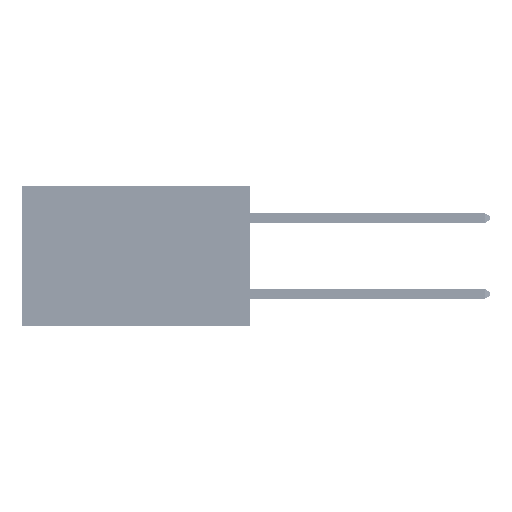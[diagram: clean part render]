
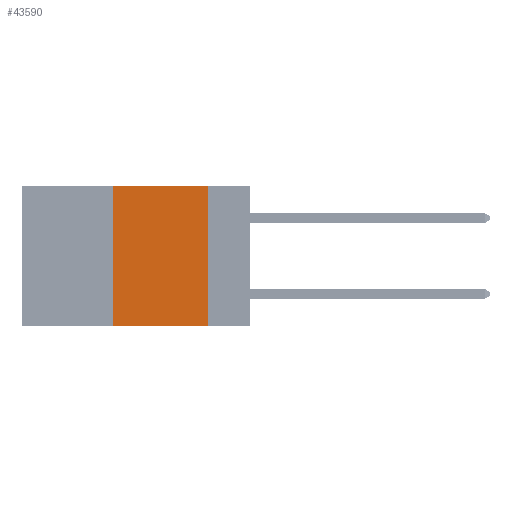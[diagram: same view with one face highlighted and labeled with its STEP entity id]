
A CAD part, left-side view. The second image highlights one B-rep face of the part: STEP entity #43590.
In plain terms, the highlighted planar face has unit normal (-1, 0, 0).
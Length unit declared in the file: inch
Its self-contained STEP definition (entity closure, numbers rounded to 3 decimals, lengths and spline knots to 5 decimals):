
#87 = VERTEX_POINT ( 'NONE', #6305 ) ;
#2628 = DIRECTION ( 'NONE',  ( 1., 0., 0. ) ) ;
#6305 = CARTESIAN_POINT ( 'NONE',  ( 0., 0.36, -0.37 ) ) ;
#7148 = LINE ( 'NONE', #38826, #11067 ) ;
#8899 = LINE ( 'NONE', #16185, #26012 ) ;
#9311 = LINE ( 'NONE', #45603, #25820 ) ;
#10166 = VERTEX_POINT ( 'NONE', #28662 ) ;
#11067 = VECTOR ( 'NONE', #35047, 39.37008 ) ;
#13826 = PLANE ( 'NONE',  #17814 ) ;
#14744 = ORIENTED_EDGE ( 'NONE', *, *, #47009, .T. ) ;
#16185 = CARTESIAN_POINT ( 'NONE',  ( 0., 0.11, 0. ) ) ;
#17814 = AXIS2_PLACEMENT_3D ( 'NONE', #18405, #2628, #21820 ) ;
#18236 = DIRECTION ( 'NONE',  ( 0., -1., 0. ) ) ;
#18269 = LINE ( 'NONE', #31185, #23751 ) ;
#18405 = CARTESIAN_POINT ( 'NONE',  ( 0., 0.6, 0. ) ) ;
#21820 = DIRECTION ( 'NONE',  ( 0., 0., -1. ) ) ;
#22657 = CARTESIAN_POINT ( 'NONE',  ( 0., 0.36, 0. ) ) ;
#22706 = CARTESIAN_POINT ( 'NONE',  ( 0., 0.11, 0. ) ) ;
#22881 = EDGE_CURVE ( 'NONE', #48929, #10166, #8899, .T. ) ;
#23751 = VECTOR ( 'NONE', #42686, 39.37008 ) ;
#25820 = VECTOR ( 'NONE', #18236, 39.37008 ) ;
#25941 = ORIENTED_EDGE ( 'NONE', *, *, #27470, .F. ) ;
#26012 = VECTOR ( 'NONE', #36666, 39.37008 ) ;
#27470 = EDGE_CURVE ( 'NONE', #87, #42415, #18269, .T. ) ;
#27716 = ORIENTED_EDGE ( 'NONE', *, *, #22881, .F. ) ;
#28662 = CARTESIAN_POINT ( 'NONE',  ( 0., 0.11, -0.37 ) ) ;
#31185 = CARTESIAN_POINT ( 'NONE',  ( 0., 0.36, 0. ) ) ;
#34156 = EDGE_LOOP ( 'NONE', ( #27716, #42161, #25941, #14744 ) ) ;
#35047 = DIRECTION ( 'NONE',  ( 0., -1., 0. ) ) ;
#36666 = DIRECTION ( 'NONE',  ( 0., 0., -1. ) ) ;
#38826 = CARTESIAN_POINT ( 'NONE',  ( 0., 0.6, -0.37 ) ) ;
#41156 = FACE_OUTER_BOUND ( 'NONE', #34156, .T. ) ;
#42161 = ORIENTED_EDGE ( 'NONE', *, *, #43551, .F. ) ;
#42415 = VERTEX_POINT ( 'NONE', #22657 ) ;
#42686 = DIRECTION ( 'NONE',  ( 0., 0., 1. ) ) ;
#43551 = EDGE_CURVE ( 'NONE', #42415, #48929, #9311, .T. ) ;
#43590 = ADVANCED_FACE ( 'NONE', ( #41156 ), #13826, .F. ) ;
#45603 = CARTESIAN_POINT ( 'NONE',  ( 0., 0.6, 0. ) ) ;
#47009 = EDGE_CURVE ( 'NONE', #87, #10166, #7148, .T. ) ;
#48929 = VERTEX_POINT ( 'NONE', #22706 ) ;
